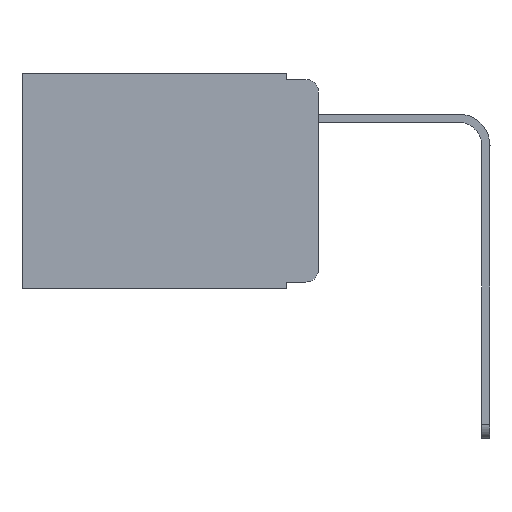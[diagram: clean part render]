
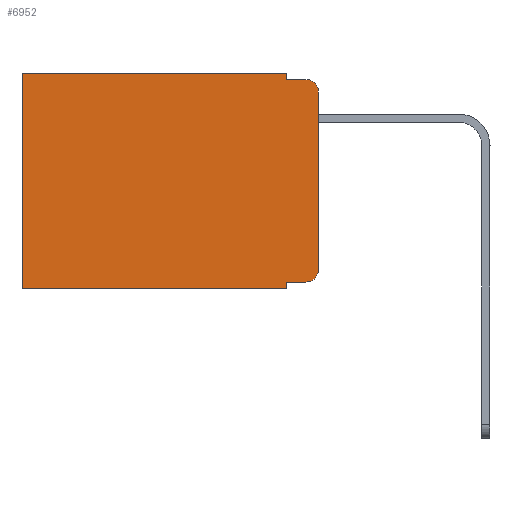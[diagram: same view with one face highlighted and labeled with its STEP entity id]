
A CAD part, left-side view. The second image highlights one B-rep face of the part: STEP entity #6952.
In plain terms, the highlighted planar face has unit normal (-1, 0, 0).
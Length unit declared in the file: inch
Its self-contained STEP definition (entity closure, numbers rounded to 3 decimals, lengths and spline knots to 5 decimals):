
#172 = LINE ( 'NONE', #12338, #2213 ) ;
#182 = VERTEX_POINT ( 'NONE', #11909 ) ;
#1129 = CARTESIAN_POINT ( 'NONE',  ( 0.298, 0., 0. ) ) ;
#1618 = EDGE_LOOP ( 'NONE', ( #19954, #8586, #12330, #2040, #11117, #7991, #3940, #14548, #14757, #15137 ) ) ;
#2040 = ORIENTED_EDGE ( 'NONE', *, *, #9770, .F. ) ;
#2066 = EDGE_CURVE ( 'NONE', #16265, #20307, #172, .T. ) ;
#2118 = CARTESIAN_POINT ( 'NONE',  ( 0.298, 0.473, 0. ) ) ;
#2213 = VECTOR ( 'NONE', #4054, 39.37008 ) ;
#2489 = CARTESIAN_POINT ( 'NONE',  ( 0.298, 0.473, 0. ) ) ;
#2567 = EDGE_CURVE ( 'NONE', #20307, #14688, #7076, .T. ) ;
#3121 = VECTOR ( 'NONE', #5066, 39.37008 ) ;
#3940 = ORIENTED_EDGE ( 'NONE', *, *, #9741, .F. ) ;
#4054 = DIRECTION ( 'NONE',  ( 0., 1., 0. ) ) ;
#4349 = VECTOR ( 'NONE', #15090, 39.37008 ) ;
#5066 = DIRECTION ( 'NONE',  ( 0., -1., 0. ) ) ;
#5178 = CIRCLE ( 'NONE', #9941, 0.02 ) ;
#5372 = CARTESIAN_POINT ( 'NONE',  ( 0.298, 0.02, -0.03 ) ) ;
#5508 = DIRECTION ( 'NONE',  ( 0., 0., -1. ) ) ;
#5746 = DIRECTION ( 'NONE',  ( 0., -1., 0. ) ) ;
#6952 = ADVANCED_FACE ( 'NONE', ( #11969 ), #19354, .F. ) ;
#7076 = LINE ( 'NONE', #2489, #10361 ) ;
#7344 = DIRECTION ( 'NONE',  ( 0., 0., -1. ) ) ;
#7470 = DIRECTION ( 'NONE',  ( 0., 0., -1. ) ) ;
#7633 = LINE ( 'NONE', #20604, #10436 ) ;
#7750 = EDGE_CURVE ( 'NONE', #182, #8611, #18970, .T. ) ;
#7843 = CARTESIAN_POINT ( 'NONE',  ( 0.298, 0.051, 0. ) ) ;
#7920 = LINE ( 'NONE', #13441, #18674 ) ;
#7991 = ORIENTED_EDGE ( 'NONE', *, *, #2567, .T. ) ;
#8586 = ORIENTED_EDGE ( 'NONE', *, *, #14011, .T. ) ;
#8611 = VERTEX_POINT ( 'NONE', #9693 ) ;
#9317 = CARTESIAN_POINT ( 'NONE',  ( 0.298, 0.473, -0.343 ) ) ;
#9428 = DIRECTION ( 'NONE',  ( 0., 0., -1. ) ) ;
#9693 = CARTESIAN_POINT ( 'NONE',  ( 0.298, 0.02, -0.333 ) ) ;
#9741 = EDGE_CURVE ( 'NONE', #14265, #14688, #18165, .T. ) ;
#9770 = EDGE_CURVE ( 'NONE', #16265, #11494, #7920, .T. ) ;
#9936 = VECTOR ( 'NONE', #12216, 39.37008 ) ;
#9941 = AXIS2_PLACEMENT_3D ( 'NONE', #5372, #17096, #5508 ) ;
#10018 = CARTESIAN_POINT ( 'NONE',  ( 0.298, 0., 0. ) ) ;
#10232 = LINE ( 'NONE', #10018, #4349 ) ;
#10361 = VECTOR ( 'NONE', #7344, 39.37008 ) ;
#10406 = EDGE_CURVE ( 'NONE', #11494, #19422, #7633, .T. ) ;
#10436 = VECTOR ( 'NONE', #5746, 39.37008 ) ;
#11117 = ORIENTED_EDGE ( 'NONE', *, *, #2066, .T. ) ;
#11494 = VERTEX_POINT ( 'NONE', #15663 ) ;
#11782 = DIRECTION ( 'NONE',  ( 0., 0., -1. ) ) ;
#11909 = CARTESIAN_POINT ( 'NONE',  ( 0.298, 0.051, -0.333 ) ) ;
#11955 = LINE ( 'NONE', #17455, #9936 ) ;
#11969 = FACE_OUTER_BOUND ( 'NONE', #1618, .T. ) ;
#12216 = DIRECTION ( 'NONE',  ( 0., 0., -1. ) ) ;
#12330 = ORIENTED_EDGE ( 'NONE', *, *, #10406, .F. ) ;
#12335 = CARTESIAN_POINT ( 'NONE',  ( 0.298, 0., -0.03 ) ) ;
#12338 = CARTESIAN_POINT ( 'NONE',  ( 0.298, 0., 0. ) ) ;
#12398 = CARTESIAN_POINT ( 'NONE',  ( 0.298, 0.02, -0.313 ) ) ;
#13090 = CARTESIAN_POINT ( 'NONE',  ( 0.298, 0., -0.343 ) ) ;
#13354 = VERTEX_POINT ( 'NONE', #12335 ) ;
#13441 = CARTESIAN_POINT ( 'NONE',  ( 0.298, 0.051, 0. ) ) ;
#14011 = EDGE_CURVE ( 'NONE', #13354, #19422, #5178, .T. ) ;
#14265 = VERTEX_POINT ( 'NONE', #20312 ) ;
#14306 = CARTESIAN_POINT ( 'NONE',  ( 0.298, 0.02, -0.01 ) ) ;
#14548 = ORIENTED_EDGE ( 'NONE', *, *, #21047, .F. ) ;
#14688 = VERTEX_POINT ( 'NONE', #9317 ) ;
#14757 = ORIENTED_EDGE ( 'NONE', *, *, #7750, .T. ) ;
#14787 = EDGE_CURVE ( 'NONE', #13354, #16068, #10232, .T. ) ;
#14941 = CARTESIAN_POINT ( 'NONE',  ( 0.298, 0.051, -0.333 ) ) ;
#15090 = DIRECTION ( 'NONE',  ( 0., 0., -1. ) ) ;
#15137 = ORIENTED_EDGE ( 'NONE', *, *, #16587, .T. ) ;
#15165 = DIRECTION ( 'NONE',  ( 0., 1., 0. ) ) ;
#15663 = CARTESIAN_POINT ( 'NONE',  ( 0.298, 0.051, -0.01 ) ) ;
#15954 = DIRECTION ( 'NONE',  ( 1., 0., 0. ) ) ;
#16068 = VERTEX_POINT ( 'NONE', #17612 ) ;
#16265 = VERTEX_POINT ( 'NONE', #7843 ) ;
#16587 = EDGE_CURVE ( 'NONE', #8611, #16068, #19887, .T. ) ;
#17096 = DIRECTION ( 'NONE',  ( -1., 0., 0. ) ) ;
#17109 = AXIS2_PLACEMENT_3D ( 'NONE', #1129, #15954, #9428 ) ;
#17455 = CARTESIAN_POINT ( 'NONE',  ( 0.298, 0.051, 0. ) ) ;
#17517 = AXIS2_PLACEMENT_3D ( 'NONE', #12398, #18917, #7470 ) ;
#17612 = CARTESIAN_POINT ( 'NONE',  ( 0.298, 0., -0.313 ) ) ;
#18165 = LINE ( 'NONE', #13090, #19947 ) ;
#18674 = VECTOR ( 'NONE', #11782, 39.37008 ) ;
#18917 = DIRECTION ( 'NONE',  ( -1., 0., 0. ) ) ;
#18970 = LINE ( 'NONE', #14941, #3121 ) ;
#19354 = PLANE ( 'NONE',  #17109 ) ;
#19422 = VERTEX_POINT ( 'NONE', #14306 ) ;
#19887 = CIRCLE ( 'NONE', #17517, 0.02 ) ;
#19947 = VECTOR ( 'NONE', #15165, 39.37008 ) ;
#19954 = ORIENTED_EDGE ( 'NONE', *, *, #14787, .F. ) ;
#20307 = VERTEX_POINT ( 'NONE', #2118 ) ;
#20312 = CARTESIAN_POINT ( 'NONE',  ( 0.298, 0.051, -0.343 ) ) ;
#20604 = CARTESIAN_POINT ( 'NONE',  ( 0.298, 0.051, -0.01 ) ) ;
#21047 = EDGE_CURVE ( 'NONE', #182, #14265, #11955, .T. ) ;
